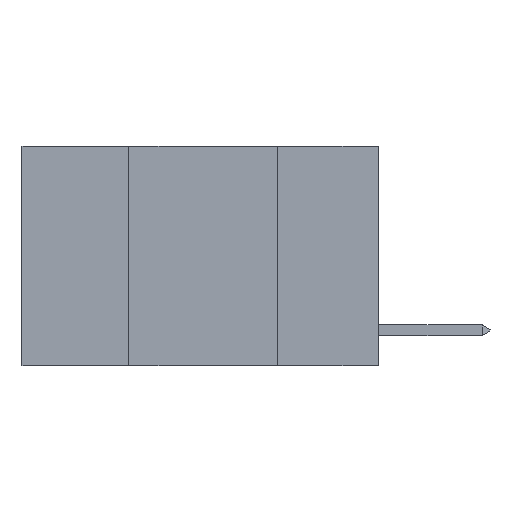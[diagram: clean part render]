
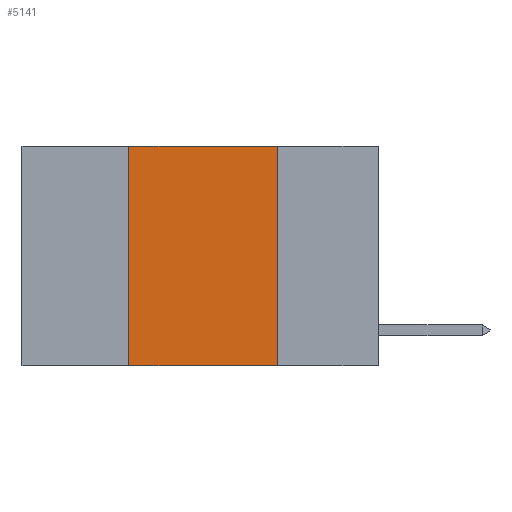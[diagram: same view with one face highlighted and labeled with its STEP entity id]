
A CAD part, left-side view. The second image highlights one B-rep face of the part: STEP entity #5141.
In plain terms, the highlighted planar face has unit normal (-1, 0, 0).
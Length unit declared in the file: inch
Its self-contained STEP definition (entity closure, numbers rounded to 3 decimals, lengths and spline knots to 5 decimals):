
#912 = VERTEX_POINT ( 'NONE', #8564 ) ;
#948 = VECTOR ( 'NONE', #12796, 39.37008 ) ;
#1160 = CARTESIAN_POINT ( 'NONE',  ( 0., 0.6, 0. ) ) ;
#1192 = ORIENTED_EDGE ( 'NONE', *, *, #15831, .F. ) ;
#1479 = FACE_OUTER_BOUND ( 'NONE', #12738, .T. ) ;
#2149 = ORIENTED_EDGE ( 'NONE', *, *, #8045, .T. ) ;
#2228 = VERTEX_POINT ( 'NONE', #10339 ) ;
#2386 = VERTEX_POINT ( 'NONE', #4587 ) ;
#2497 = CARTESIAN_POINT ( 'NONE',  ( 0., 0.6, 0. ) ) ;
#2623 = PLANE ( 'NONE',  #15501 ) ;
#2724 = CARTESIAN_POINT ( 'NONE',  ( 0., 0.17, 0. ) ) ;
#3222 = CARTESIAN_POINT ( 'NONE',  ( 0., 0.6, -0.37 ) ) ;
#3568 = VECTOR ( 'NONE', #11333, 39.37008 ) ;
#4030 = LINE ( 'NONE', #9869, #3568 ) ;
#4198 = DIRECTION ( 'NONE',  ( 0., 0., -1. ) ) ;
#4504 = LINE ( 'NONE', #2497, #948 ) ;
#4587 = CARTESIAN_POINT ( 'NONE',  ( 0., 0.17, 0. ) ) ;
#4728 = ORIENTED_EDGE ( 'NONE', *, *, #16435, .F. ) ;
#5141 = ADVANCED_FACE ( 'NONE', ( #1479 ), #2623, .F. ) ;
#8045 = EDGE_CURVE ( 'NONE', #2228, #11584, #10454, .T. ) ;
#8564 = CARTESIAN_POINT ( 'NONE',  ( 0., 0.42, 0. ) ) ;
#8804 = VECTOR ( 'NONE', #15983, 39.37008 ) ;
#9410 = CARTESIAN_POINT ( 'NONE',  ( 0., 0.17, -0.37 ) ) ;
#9869 = CARTESIAN_POINT ( 'NONE',  ( 0., 0.42, 0. ) ) ;
#10339 = CARTESIAN_POINT ( 'NONE',  ( 0., 0.42, -0.37 ) ) ;
#10454 = LINE ( 'NONE', #3222, #17753 ) ;
#11333 = DIRECTION ( 'NONE',  ( 0., 0., 1. ) ) ;
#11584 = VERTEX_POINT ( 'NONE', #9410 ) ;
#12738 = EDGE_LOOP ( 'NONE', ( #15976, #4728, #1192, #2149 ) ) ;
#12796 = DIRECTION ( 'NONE',  ( 0., -1., 0. ) ) ;
#12998 = DIRECTION ( 'NONE',  ( 1., 0., 0. ) ) ;
#14999 = DIRECTION ( 'NONE',  ( 0., -1., 0. ) ) ;
#15501 = AXIS2_PLACEMENT_3D ( 'NONE', #1160, #12998, #4198 ) ;
#15831 = EDGE_CURVE ( 'NONE', #2228, #912, #4030, .T. ) ;
#15976 = ORIENTED_EDGE ( 'NONE', *, *, #17866, .F. ) ;
#15983 = DIRECTION ( 'NONE',  ( 0., 0., -1. ) ) ;
#16435 = EDGE_CURVE ( 'NONE', #912, #2386, #4504, .T. ) ;
#16607 = LINE ( 'NONE', #2724, #8804 ) ;
#17753 = VECTOR ( 'NONE', #14999, 39.37008 ) ;
#17866 = EDGE_CURVE ( 'NONE', #2386, #11584, #16607, .T. ) ;
